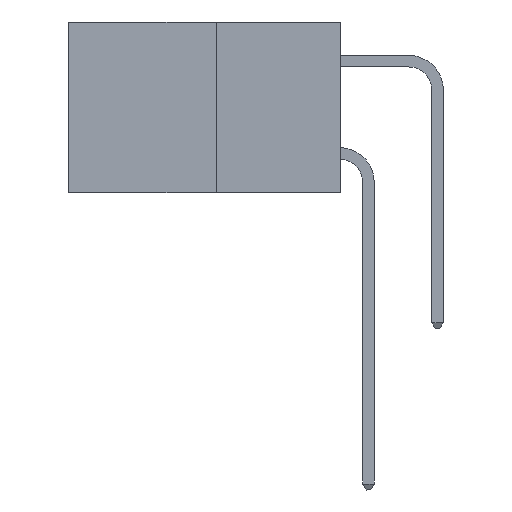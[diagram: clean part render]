
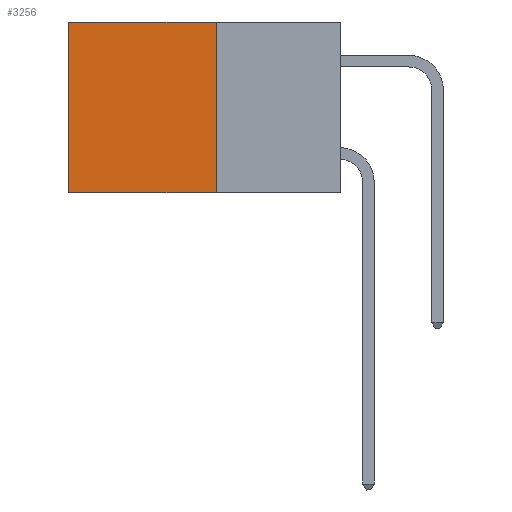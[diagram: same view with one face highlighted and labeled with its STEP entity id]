
A CAD part, left-side view. The second image highlights one B-rep face of the part: STEP entity #3256.
In plain terms, the highlighted planar face has unit normal (-1, 0, 0).
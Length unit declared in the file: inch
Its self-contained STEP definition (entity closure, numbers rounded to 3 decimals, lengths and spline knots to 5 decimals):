
#162 = VERTEX_POINT ( 'NONE', #6722 ) ;
#372 = EDGE_CURVE ( 'NONE', #9404, #7811, #7238, .T. ) ;
#664 = EDGE_LOOP ( 'NONE', ( #6933, #6364, #8630, #8056 ) ) ;
#828 = CARTESIAN_POINT ( 'NONE',  ( 0.277, 0.27, -0.37 ) ) ;
#1401 = PLANE ( 'NONE',  #4187 ) ;
#1419 = VERTEX_POINT ( 'NONE', #7984 ) ;
#2123 = DIRECTION ( 'NONE',  ( 0., 1., 0. ) ) ;
#2293 = CARTESIAN_POINT ( 'NONE',  ( 0.277, 0.27, 0. ) ) ;
#2395 = EDGE_CURVE ( 'NONE', #162, #7811, #9234, .T. ) ;
#2548 = CARTESIAN_POINT ( 'NONE',  ( 0.277, 0.27, -0.37 ) ) ;
#2845 = EDGE_CURVE ( 'NONE', #1419, #9404, #4889, .T. ) ;
#2964 = VECTOR ( 'NONE', #3263, 39.37008 ) ;
#3256 = ADVANCED_FACE ( 'NONE', ( #8544 ), #1401, .F. ) ;
#3263 = DIRECTION ( 'NONE',  ( 0., 0., -1. ) ) ;
#3273 = CARTESIAN_POINT ( 'NONE',  ( 0.277, 0.27, -0.37 ) ) ;
#3946 = DIRECTION ( 'NONE',  ( 0., 0., -1. ) ) ;
#4187 = AXIS2_PLACEMENT_3D ( 'NONE', #828, #5268, #4484 ) ;
#4484 = DIRECTION ( 'NONE',  ( 0., 0., -1. ) ) ;
#4759 = VECTOR ( 'NONE', #2123, 39.37008 ) ;
#4889 = LINE ( 'NONE', #2548, #2964 ) ;
#5050 = VECTOR ( 'NONE', #6391, 39.37008 ) ;
#5124 = VECTOR ( 'NONE', #3946, 39.37008 ) ;
#5268 = DIRECTION ( 'NONE',  ( 1., 0., 0. ) ) ;
#6364 = ORIENTED_EDGE ( 'NONE', *, *, #372, .F. ) ;
#6391 = DIRECTION ( 'NONE',  ( 0., 1., 0. ) ) ;
#6722 = CARTESIAN_POINT ( 'NONE',  ( 0.277, 0.59, 0. ) ) ;
#6724 = LINE ( 'NONE', #2293, #4759 ) ;
#6768 = EDGE_CURVE ( 'NONE', #1419, #162, #6724, .T. ) ;
#6933 = ORIENTED_EDGE ( 'NONE', *, *, #2395, .T. ) ;
#7024 = CARTESIAN_POINT ( 'NONE',  ( 0.277, 0.59, -0.37 ) ) ;
#7238 = LINE ( 'NONE', #7832, #5050 ) ;
#7800 = CARTESIAN_POINT ( 'NONE',  ( 0.277, 0.59, -0.37 ) ) ;
#7811 = VERTEX_POINT ( 'NONE', #7024 ) ;
#7832 = CARTESIAN_POINT ( 'NONE',  ( 0.277, 0.27, -0.37 ) ) ;
#7984 = CARTESIAN_POINT ( 'NONE',  ( 0.277, 0.27, 0. ) ) ;
#8056 = ORIENTED_EDGE ( 'NONE', *, *, #6768, .T. ) ;
#8544 = FACE_OUTER_BOUND ( 'NONE', #664, .T. ) ;
#8630 = ORIENTED_EDGE ( 'NONE', *, *, #2845, .F. ) ;
#9234 = LINE ( 'NONE', #7800, #5124 ) ;
#9404 = VERTEX_POINT ( 'NONE', #3273 ) ;
